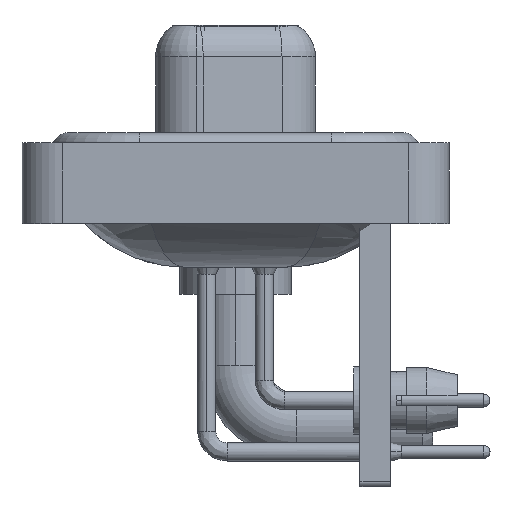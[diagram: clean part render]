
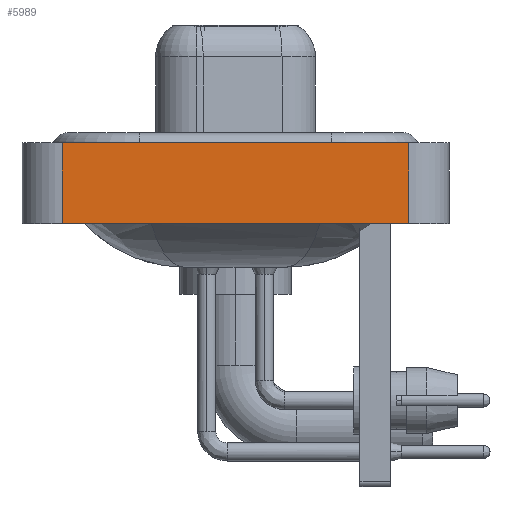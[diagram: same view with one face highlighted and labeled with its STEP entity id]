
A CAD part, left-side view. The second image highlights one B-rep face of the part: STEP entity #5989.
In plain terms, the highlighted planar face has unit normal (-1, 0, 0).
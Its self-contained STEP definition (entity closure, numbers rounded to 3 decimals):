
#425 = CARTESIAN_POINT ( 'NONE',  ( -7.35, -8.55, -3.6 ) ) ;
#622 = PLANE ( 'NONE',  #14105 ) ;
#845 = CARTESIAN_POINT ( 'NONE',  ( -7.35, -8.55, -3.6 ) ) ;
#986 = VERTEX_POINT ( 'NONE', #21352 ) ;
#2497 = CARTESIAN_POINT ( 'NONE',  ( -7.35, -8.55, -3.6 ) ) ;
#3185 = LINE ( 'NONE', #845, #7191 ) ;
#4106 = LINE ( 'NONE', #21327, #14309 ) ;
#4948 = DIRECTION ( 'NONE',  ( 0., 0., 1. ) ) ;
#5082 = CARTESIAN_POINT ( 'NONE',  ( -7.35, 8.55, -3.6 ) ) ;
#5989 = ADVANCED_FACE ( 'NONE', ( #18983 ), #622, .T. ) ;
#7174 = EDGE_LOOP ( 'NONE', ( #7980, #16738, #23456, #12417 ) ) ;
#7191 = VECTOR ( 'NONE', #21369, 1000. ) ;
#7429 = DIRECTION ( 'NONE',  ( 0., 0., 1. ) ) ;
#7980 = ORIENTED_EDGE ( 'NONE', *, *, #25364, .T. ) ;
#11650 = LINE ( 'NONE', #425, #15873 ) ;
#12417 = ORIENTED_EDGE ( 'NONE', *, *, #23957, .T. ) ;
#12968 = DIRECTION ( 'NONE',  ( 0., -1., 0. ) ) ;
#13809 = VERTEX_POINT ( 'NONE', #2497 ) ;
#14105 = AXIS2_PLACEMENT_3D ( 'NONE', #25154, #16506, #20889 ) ;
#14309 = VECTOR ( 'NONE', #12968, 1000. ) ;
#14462 = CARTESIAN_POINT ( 'NONE',  ( -7.35, 8.55, 0.4 ) ) ;
#15372 = EDGE_CURVE ( 'NONE', #15942, #26725, #25234, .T. ) ;
#15873 = VECTOR ( 'NONE', #7429, 1000. ) ;
#15942 = VERTEX_POINT ( 'NONE', #16970 ) ;
#16506 = DIRECTION ( 'NONE',  ( -1., 0., 0. ) ) ;
#16738 = ORIENTED_EDGE ( 'NONE', *, *, #18957, .F. ) ;
#16970 = CARTESIAN_POINT ( 'NONE',  ( -7.35, 8.55, -3.6 ) ) ;
#18957 = EDGE_CURVE ( 'NONE', #26725, #986, #4106, .T. ) ;
#18983 = FACE_OUTER_BOUND ( 'NONE', #7174, .T. ) ;
#19348 = VECTOR ( 'NONE', #4948, 1000. ) ;
#20889 = DIRECTION ( 'NONE',  ( 0., 0., 1. ) ) ;
#21327 = CARTESIAN_POINT ( 'NONE',  ( -7.35, -8.55, 0.4 ) ) ;
#21352 = CARTESIAN_POINT ( 'NONE',  ( -7.35, -8.55, 0.4 ) ) ;
#21369 = DIRECTION ( 'NONE',  ( 0., -1., 0. ) ) ;
#23456 = ORIENTED_EDGE ( 'NONE', *, *, #15372, .F. ) ;
#23957 = EDGE_CURVE ( 'NONE', #15942, #13809, #3185, .T. ) ;
#25154 = CARTESIAN_POINT ( 'NONE',  ( -7.35, -8.55, -3.6 ) ) ;
#25234 = LINE ( 'NONE', #5082, #19348 ) ;
#25364 = EDGE_CURVE ( 'NONE', #13809, #986, #11650, .T. ) ;
#26725 = VERTEX_POINT ( 'NONE', #14462 ) ;
